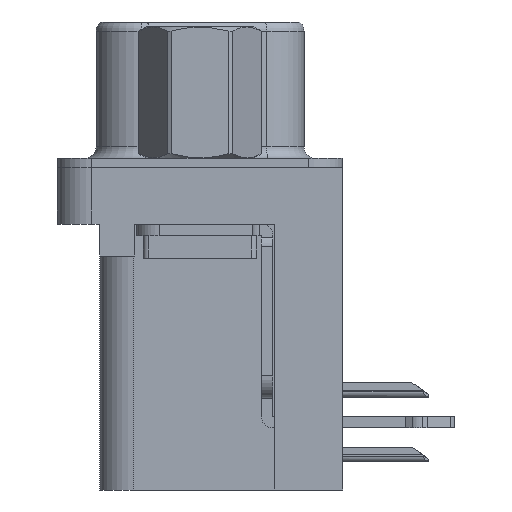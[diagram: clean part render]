
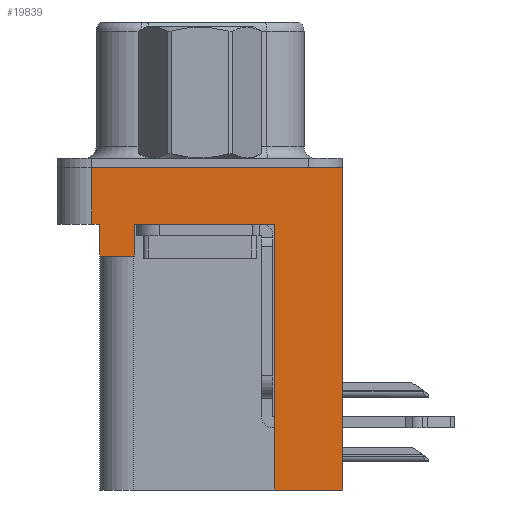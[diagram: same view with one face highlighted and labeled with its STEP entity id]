
A CAD part, left-side view. The second image highlights one B-rep face of the part: STEP entity #19839.
In plain terms, the highlighted planar face has unit normal (-1, 0, 0).
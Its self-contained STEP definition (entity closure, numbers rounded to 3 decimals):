
#165 = CARTESIAN_POINT ( 'NONE',  ( -2.91, -6.275, -14.2 ) ) ;
#329 = VECTOR ( 'NONE', #2552, 1000. ) ;
#637 = VECTOR ( 'NONE', #27429, 1000. ) ;
#1174 = VECTOR ( 'NONE', #20215, 1000. ) ;
#1763 = VERTEX_POINT ( 'NONE', #5032 ) ;
#2328 = VERTEX_POINT ( 'NONE', #14752 ) ;
#2525 = ORIENTED_EDGE ( 'NONE', *, *, #21424, .F. ) ;
#2552 = DIRECTION ( 'NONE',  ( 0., 1., 0. ) ) ;
#2890 = VECTOR ( 'NONE', #26293, 1000. ) ;
#3192 = CARTESIAN_POINT ( 'NONE',  ( -2.91, 4.775, -2.5 ) ) ;
#4651 = LINE ( 'NONE', #10044, #27556 ) ;
#4709 = CARTESIAN_POINT ( 'NONE',  ( -2.91, -3.295, -14.2 ) ) ;
#5032 = CARTESIAN_POINT ( 'NONE',  ( -2.91, 4.775, 0. ) ) ;
#5310 = LINE ( 'NONE', #3192, #9226 ) ;
#5618 = VERTEX_POINT ( 'NONE', #6062 ) ;
#6062 = CARTESIAN_POINT ( 'NONE',  ( -2.91, 4.425, -2.5 ) ) ;
#6768 = ORIENTED_EDGE ( 'NONE', *, *, #20595, .F. ) ;
#8811 = DIRECTION ( 'NONE',  ( -1., 0., 0. ) ) ;
#8841 = CARTESIAN_POINT ( 'NONE',  ( -2.91, 4.425, -3.9 ) ) ;
#8920 = VERTEX_POINT ( 'NONE', #9078 ) ;
#9033 = VECTOR ( 'NONE', #15573, 1000. ) ;
#9078 = CARTESIAN_POINT ( 'NONE',  ( -2.91, -3.295, -14.2 ) ) ;
#9148 = VERTEX_POINT ( 'NONE', #22479 ) ;
#9226 = VECTOR ( 'NONE', #12989, 1000. ) ;
#9404 = VERTEX_POINT ( 'NONE', #165 ) ;
#9866 = EDGE_CURVE ( 'NONE', #16670, #5618, #28069, .T. ) ;
#9992 = CARTESIAN_POINT ( 'NONE',  ( -2.91, 2.895, -3.9 ) ) ;
#10044 = CARTESIAN_POINT ( 'NONE',  ( -2.91, -6.275, -2.5 ) ) ;
#10088 = EDGE_LOOP ( 'NONE', ( #21358, #23853, #29478, #10355, #26907, #29214, #29626, #6768, #2525, #10279 ) ) ;
#10279 = ORIENTED_EDGE ( 'NONE', *, *, #22649, .T. ) ;
#10355 = ORIENTED_EDGE ( 'NONE', *, *, #9866, .F. ) ;
#11669 = EDGE_CURVE ( 'NONE', #2328, #1763, #5310, .T. ) ;
#12657 = VECTOR ( 'NONE', #28800, 1000. ) ;
#12690 = CARTESIAN_POINT ( 'NONE',  ( -2.91, -6.275, 0. ) ) ;
#12989 = DIRECTION ( 'NONE',  ( 0., 0., 1. ) ) ;
#14752 = CARTESIAN_POINT ( 'NONE',  ( -2.91, 4.775, -2.5 ) ) ;
#15435 = VERTEX_POINT ( 'NONE', #22831 ) ;
#15573 = DIRECTION ( 'NONE',  ( 0., -1., 0. ) ) ;
#16317 = LINE ( 'NONE', #23676, #2890 ) ;
#16396 = CARTESIAN_POINT ( 'NONE',  ( -2.91, -6.275, -2.5 ) ) ;
#16670 = VERTEX_POINT ( 'NONE', #8841 ) ;
#17441 = CARTESIAN_POINT ( 'NONE',  ( -2.91, -3.295, -2.5 ) ) ;
#19503 = VERTEX_POINT ( 'NONE', #12690 ) ;
#19839 = ADVANCED_FACE ( 'NONE', ( #24176 ), #28747, .T. ) ;
#19975 = DIRECTION ( 'NONE',  ( 0., 0., 1. ) ) ;
#20215 = DIRECTION ( 'NONE',  ( 0., 0., 1. ) ) ;
#20399 = CARTESIAN_POINT ( 'NONE',  ( -2.91, 4.425, -3.9 ) ) ;
#20595 = EDGE_CURVE ( 'NONE', #8920, #28775, #20687, .T. ) ;
#20687 = LINE ( 'NONE', #27714, #1174 ) ;
#21184 = EDGE_CURVE ( 'NONE', #1763, #19503, #28151, .T. ) ;
#21358 = ORIENTED_EDGE ( 'NONE', *, *, #21184, .F. ) ;
#21424 = EDGE_CURVE ( 'NONE', #9404, #8920, #30205, .T. ) ;
#21869 = LINE ( 'NONE', #24955, #329 ) ;
#22421 = LINE ( 'NONE', #9992, #22886 ) ;
#22470 = DIRECTION ( 'NONE',  ( 0., -1., 0. ) ) ;
#22479 = CARTESIAN_POINT ( 'NONE',  ( -2.91, 2.895, -3.9 ) ) ;
#22649 = EDGE_CURVE ( 'NONE', #9404, #19503, #28963, .T. ) ;
#22784 = CARTESIAN_POINT ( 'NONE',  ( -2.91, -6.275, 0. ) ) ;
#22831 = CARTESIAN_POINT ( 'NONE',  ( -2.91, 2.895, -2.5 ) ) ;
#22886 = VECTOR ( 'NONE', #19975, 1000. ) ;
#23178 = DIRECTION ( 'NONE',  ( 0., 0., 1. ) ) ;
#23676 = CARTESIAN_POINT ( 'NONE',  ( -2.91, -6.275, -2.5 ) ) ;
#23853 = ORIENTED_EDGE ( 'NONE', *, *, #11669, .F. ) ;
#24176 = FACE_OUTER_BOUND ( 'NONE', #10088, .T. ) ;
#24955 = CARTESIAN_POINT ( 'NONE',  ( -2.91, 4.425, -3.9 ) ) ;
#25901 = EDGE_CURVE ( 'NONE', #2328, #5618, #16317, .T. ) ;
#26144 = DIRECTION ( 'NONE',  ( 0., 0., 1. ) ) ;
#26293 = DIRECTION ( 'NONE',  ( 0., -1., 0. ) ) ;
#26907 = ORIENTED_EDGE ( 'NONE', *, *, #28732, .F. ) ;
#27429 = DIRECTION ( 'NONE',  ( 0., 1., 0. ) ) ;
#27556 = VECTOR ( 'NONE', #22470, 1000. ) ;
#27714 = CARTESIAN_POINT ( 'NONE',  ( -2.91, -3.295, -14.2 ) ) ;
#28069 = LINE ( 'NONE', #20399, #29014 ) ;
#28151 = LINE ( 'NONE', #22784, #9033 ) ;
#28732 = EDGE_CURVE ( 'NONE', #9148, #16670, #21869, .T. ) ;
#28747 = PLANE ( 'NONE',  #30888 ) ;
#28775 = VERTEX_POINT ( 'NONE', #17441 ) ;
#28800 = DIRECTION ( 'NONE',  ( 0., 0., 1. ) ) ;
#28963 = LINE ( 'NONE', #16396, #12657 ) ;
#29014 = VECTOR ( 'NONE', #23178, 1000. ) ;
#29214 = ORIENTED_EDGE ( 'NONE', *, *, #31074, .T. ) ;
#29478 = ORIENTED_EDGE ( 'NONE', *, *, #25901, .T. ) ;
#29626 = ORIENTED_EDGE ( 'NONE', *, *, #30673, .T. ) ;
#30205 = LINE ( 'NONE', #4709, #637 ) ;
#30673 = EDGE_CURVE ( 'NONE', #15435, #28775, #4651, .T. ) ;
#30888 = AXIS2_PLACEMENT_3D ( 'NONE', #31352, #8811, #26144 ) ;
#31074 = EDGE_CURVE ( 'NONE', #9148, #15435, #22421, .T. ) ;
#31352 = CARTESIAN_POINT ( 'NONE',  ( -2.91, -6.275, -2.5 ) ) ;
